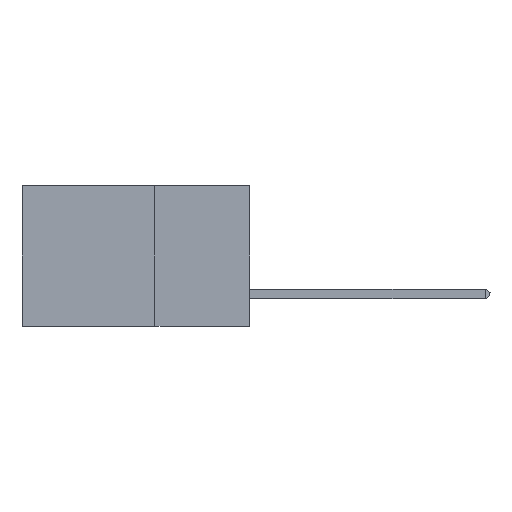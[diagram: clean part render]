
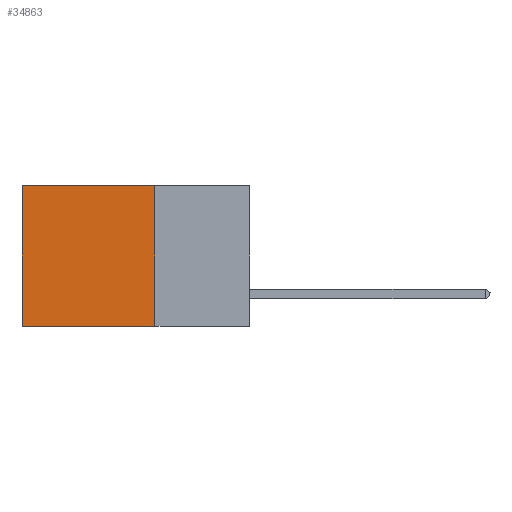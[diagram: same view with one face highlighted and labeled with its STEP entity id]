
A CAD part, left-side view. The second image highlights one B-rep face of the part: STEP entity #34863.
In plain terms, the highlighted planar face has unit normal (-1, 0, 0).
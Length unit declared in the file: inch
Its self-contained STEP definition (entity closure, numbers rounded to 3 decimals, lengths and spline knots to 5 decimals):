
#2420 = EDGE_CURVE ( 'NONE', #12811, #7146, #10709, .T. ) ;
#2421 = VECTOR ( 'NONE', #33538, 39.37008 ) ;
#4400 = CARTESIAN_POINT ( 'NONE',  ( 0.2875, 0.6, 0. ) ) ;
#6117 = ORIENTED_EDGE ( 'NONE', *, *, #2420, .T. ) ;
#6208 = CARTESIAN_POINT ( 'NONE',  ( 0.2875, 0.25, 0. ) ) ;
#7146 = VERTEX_POINT ( 'NONE', #15733 ) ;
#7448 = CARTESIAN_POINT ( 'NONE',  ( 0.2875, 0.25, -0.37 ) ) ;
#9531 = DIRECTION ( 'NONE',  ( 0., 0., -1. ) ) ;
#9792 = CARTESIAN_POINT ( 'NONE',  ( 0.2875, 0.25, 0. ) ) ;
#9915 = DIRECTION ( 'NONE',  ( 1., 0., 0. ) ) ;
#10257 = VECTOR ( 'NONE', #26890, 39.37008 ) ;
#10601 = VERTEX_POINT ( 'NONE', #7448 ) ;
#10709 = LINE ( 'NONE', #22253, #2421 ) ;
#11584 = DIRECTION ( 'NONE',  ( 0., 1., 0. ) ) ;
#11732 = DIRECTION ( 'NONE',  ( 0., 0., -1. ) ) ;
#12422 = LINE ( 'NONE', #6208, #10257 ) ;
#12811 = VERTEX_POINT ( 'NONE', #4400 ) ;
#14272 = VECTOR ( 'NONE', #11584, 39.37008 ) ;
#15733 = CARTESIAN_POINT ( 'NONE',  ( 0.2875, 0.6, -0.37 ) ) ;
#16841 = ORIENTED_EDGE ( 'NONE', *, *, #32882, .F. ) ;
#17749 = LINE ( 'NONE', #25546, #14272 ) ;
#18601 = VECTOR ( 'NONE', #11732, 39.37008 ) ;
#20031 = ORIENTED_EDGE ( 'NONE', *, *, #25613, .T. ) ;
#20726 = ORIENTED_EDGE ( 'NONE', *, *, #22809, .F. ) ;
#21287 = CARTESIAN_POINT ( 'NONE',  ( 0.2875, 0.25, 0. ) ) ;
#22253 = CARTESIAN_POINT ( 'NONE',  ( 0.2875, 0.6, 0. ) ) ;
#22809 = EDGE_CURVE ( 'NONE', #10601, #7146, #17749, .T. ) ;
#23139 = FACE_OUTER_BOUND ( 'NONE', #27937, .T. ) ;
#25546 = CARTESIAN_POINT ( 'NONE',  ( 0.2875, 0.25, -0.37 ) ) ;
#25613 = EDGE_CURVE ( 'NONE', #32511, #12811, #12422, .T. ) ;
#25931 = LINE ( 'NONE', #28305, #18601 ) ;
#26890 = DIRECTION ( 'NONE',  ( 0., 1., 0. ) ) ;
#27937 = EDGE_LOOP ( 'NONE', ( #6117, #20726, #16841, #20031 ) ) ;
#28305 = CARTESIAN_POINT ( 'NONE',  ( 0.2875, 0.25, 0. ) ) ;
#31859 = PLANE ( 'NONE',  #33689 ) ;
#32511 = VERTEX_POINT ( 'NONE', #21287 ) ;
#32882 = EDGE_CURVE ( 'NONE', #32511, #10601, #25931, .T. ) ;
#33538 = DIRECTION ( 'NONE',  ( 0., 0., -1. ) ) ;
#33689 = AXIS2_PLACEMENT_3D ( 'NONE', #9792, #9915, #9531 ) ;
#34863 = ADVANCED_FACE ( 'NONE', ( #23139 ), #31859, .F. ) ;
